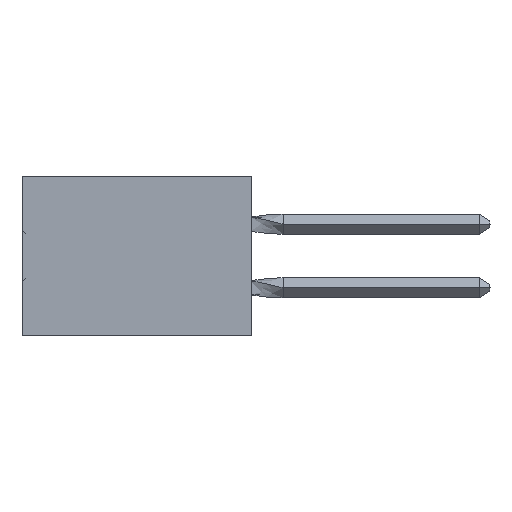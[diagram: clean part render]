
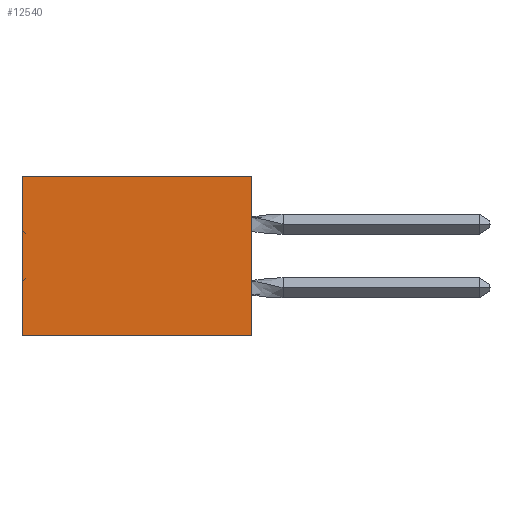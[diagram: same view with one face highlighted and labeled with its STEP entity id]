
A CAD part, left-side view. The second image highlights one B-rep face of the part: STEP entity #12540.
In plain terms, the highlighted planar face has unit normal (-1, 0, 0).
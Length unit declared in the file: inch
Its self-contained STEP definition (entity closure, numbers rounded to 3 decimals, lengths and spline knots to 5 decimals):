
#482 = DIRECTION ( 'NONE',  ( 1., 0., 0. ) ) ;
#955 = VECTOR ( 'NONE', #4345, 39.37008 ) ;
#3197 = VERTEX_POINT ( 'NONE', #27894 ) ;
#4345 = DIRECTION ( 'NONE',  ( 0., 1., 0. ) ) ;
#6445 = VECTOR ( 'NONE', #12578, 39.37008 ) ;
#6582 = DIRECTION ( 'NONE',  ( 0., 1., 0. ) ) ;
#7771 = AXIS2_PLACEMENT_3D ( 'NONE', #54901, #482, #22624 ) ;
#10258 = LINE ( 'NONE', #15063, #36661 ) ;
#12540 = ADVANCED_FACE ( 'NONE', ( #17068 ), #22810, .F. ) ;
#12578 = DIRECTION ( 'NONE',  ( 0., 0., -1. ) ) ;
#13419 = VERTEX_POINT ( 'NONE', #44266 ) ;
#13765 = ORIENTED_EDGE ( 'NONE', *, *, #26813, .T. ) ;
#13894 = EDGE_LOOP ( 'NONE', ( #13765, #47567, #48420, #58572 ) ) ;
#14633 = CARTESIAN_POINT ( 'NONE',  ( 0.305, 0., 0. ) ) ;
#15063 = CARTESIAN_POINT ( 'NONE',  ( 0.305, 0., -0.5 ) ) ;
#17068 = FACE_OUTER_BOUND ( 'NONE', #13894, .T. ) ;
#18049 = VECTOR ( 'NONE', #6582, 39.37008 ) ;
#22624 = DIRECTION ( 'NONE',  ( 0., 0., -1. ) ) ;
#22810 = PLANE ( 'NONE',  #7771 ) ;
#25632 = EDGE_CURVE ( 'NONE', #44760, #13419, #10258, .T. ) ;
#26668 = LINE ( 'NONE', #31142, #955 ) ;
#26813 = EDGE_CURVE ( 'NONE', #28347, #3197, #48658, .T. ) ;
#27894 = CARTESIAN_POINT ( 'NONE',  ( 0.305, 0.72, -0.5 ) ) ;
#28347 = VERTEX_POINT ( 'NONE', #55041 ) ;
#31142 = CARTESIAN_POINT ( 'NONE',  ( 0.305, 0., -0.5 ) ) ;
#32763 = EDGE_CURVE ( 'NONE', #13419, #3197, #26668, .T. ) ;
#35532 = CARTESIAN_POINT ( 'NONE',  ( 0.305, 0.72, -0.5 ) ) ;
#36661 = VECTOR ( 'NONE', #52794, 39.37008 ) ;
#42977 = CARTESIAN_POINT ( 'NONE',  ( 0.305, 0., 0. ) ) ;
#43933 = EDGE_CURVE ( 'NONE', #44760, #28347, #47432, .T. ) ;
#44266 = CARTESIAN_POINT ( 'NONE',  ( 0.305, 0., -0.5 ) ) ;
#44760 = VERTEX_POINT ( 'NONE', #14633 ) ;
#47432 = LINE ( 'NONE', #42977, #18049 ) ;
#47567 = ORIENTED_EDGE ( 'NONE', *, *, #32763, .F. ) ;
#48420 = ORIENTED_EDGE ( 'NONE', *, *, #25632, .F. ) ;
#48658 = LINE ( 'NONE', #35532, #6445 ) ;
#52794 = DIRECTION ( 'NONE',  ( 0., 0., -1. ) ) ;
#54901 = CARTESIAN_POINT ( 'NONE',  ( 0.305, 0., -0.5 ) ) ;
#55041 = CARTESIAN_POINT ( 'NONE',  ( 0.305, 0.72, 0. ) ) ;
#58572 = ORIENTED_EDGE ( 'NONE', *, *, #43933, .T. ) ;
